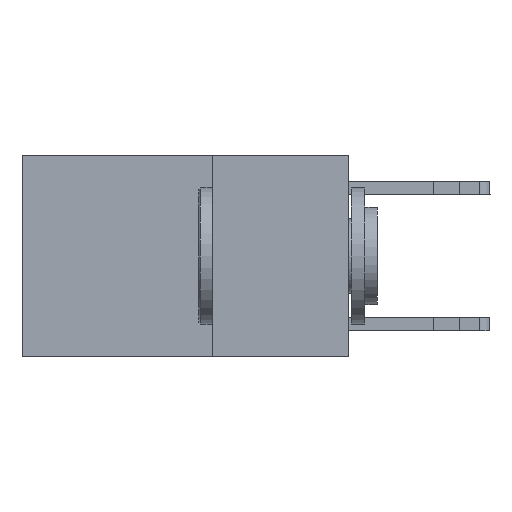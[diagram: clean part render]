
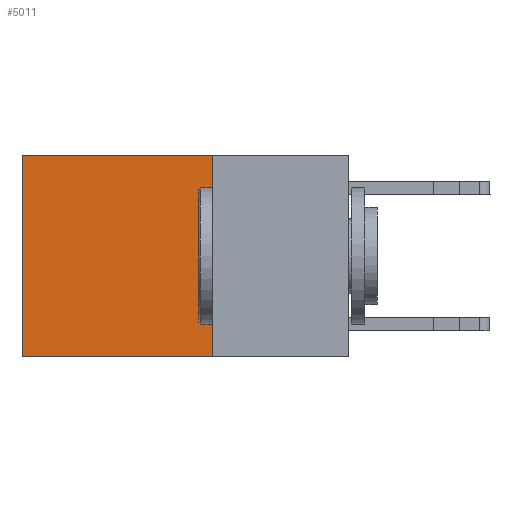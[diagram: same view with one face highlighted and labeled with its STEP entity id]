
A CAD part, left-side view. The second image highlights one B-rep face of the part: STEP entity #5011.
In plain terms, the highlighted planar face has unit normal (-1, 0, 0).
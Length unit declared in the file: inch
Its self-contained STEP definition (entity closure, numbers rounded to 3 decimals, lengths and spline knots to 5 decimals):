
#313 = VECTOR ( 'NONE', #9529, 39.37008 ) ;
#770 = FACE_OUTER_BOUND ( 'NONE', #10903, .T. ) ;
#949 = LINE ( 'NONE', #6514, #7654 ) ;
#998 = ORIENTED_EDGE ( 'NONE', *, *, #10585, .T. ) ;
#1759 = CARTESIAN_POINT ( 'NONE',  ( 0.2625, 0.25, 0. ) ) ;
#2742 = VECTOR ( 'NONE', #13200, 39.37008 ) ;
#3056 = CARTESIAN_POINT ( 'NONE',  ( 0.2625, 0.6, 0. ) ) ;
#3129 = LINE ( 'NONE', #1759, #2742 ) ;
#4147 = VECTOR ( 'NONE', #11907, 39.37008 ) ;
#4239 = VERTEX_POINT ( 'NONE', #11874 ) ;
#5011 = ADVANCED_FACE ( 'NONE', ( #770 ), #15869, .F. ) ;
#6155 = VERTEX_POINT ( 'NONE', #14226 ) ;
#6514 = CARTESIAN_POINT ( 'NONE',  ( 0.2625, 0.25, 0. ) ) ;
#6794 = CARTESIAN_POINT ( 'NONE',  ( 0.2625, 0.25, -0.37 ) ) ;
#7611 = DIRECTION ( 'NONE',  ( 1., 0., 0. ) ) ;
#7654 = VECTOR ( 'NONE', #9151, 39.37008 ) ;
#7804 = EDGE_CURVE ( 'NONE', #4239, #6155, #13759, .T. ) ;
#8766 = ORIENTED_EDGE ( 'NONE', *, *, #10054, .T. ) ;
#8894 = DIRECTION ( 'NONE',  ( 0., 0., -1. ) ) ;
#9151 = DIRECTION ( 'NONE',  ( 0., 0., -1. ) ) ;
#9189 = AXIS2_PLACEMENT_3D ( 'NONE', #13031, #7611, #8894 ) ;
#9529 = DIRECTION ( 'NONE',  ( 0., 1., 0. ) ) ;
#10054 = EDGE_CURVE ( 'NONE', #12164, #6155, #15607, .T. ) ;
#10357 = ORIENTED_EDGE ( 'NONE', *, *, #7804, .F. ) ;
#10585 = EDGE_CURVE ( 'NONE', #15949, #12164, #3129, .T. ) ;
#10903 = EDGE_LOOP ( 'NONE', ( #8766, #10357, #14119, #998 ) ) ;
#11064 = CARTESIAN_POINT ( 'NONE',  ( 0.2625, 0.6, 0. ) ) ;
#11874 = CARTESIAN_POINT ( 'NONE',  ( 0.2625, 0.25, -0.37 ) ) ;
#11907 = DIRECTION ( 'NONE',  ( 0., 0., -1. ) ) ;
#12164 = VERTEX_POINT ( 'NONE', #11064 ) ;
#13031 = CARTESIAN_POINT ( 'NONE',  ( 0.2625, 0.25, 0. ) ) ;
#13200 = DIRECTION ( 'NONE',  ( 0., 1., 0. ) ) ;
#13759 = LINE ( 'NONE', #6794, #313 ) ;
#14119 = ORIENTED_EDGE ( 'NONE', *, *, #15976, .F. ) ;
#14226 = CARTESIAN_POINT ( 'NONE',  ( 0.2625, 0.6, -0.37 ) ) ;
#15607 = LINE ( 'NONE', #3056, #4147 ) ;
#15869 = PLANE ( 'NONE',  #9189 ) ;
#15949 = VERTEX_POINT ( 'NONE', #16237 ) ;
#15976 = EDGE_CURVE ( 'NONE', #15949, #4239, #949, .T. ) ;
#16237 = CARTESIAN_POINT ( 'NONE',  ( 0.2625, 0.25, 0. ) ) ;
